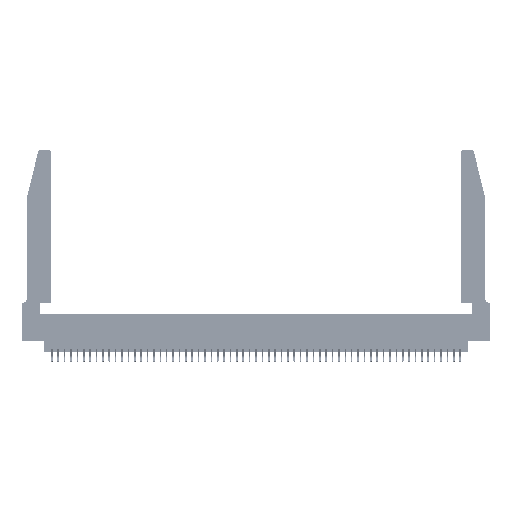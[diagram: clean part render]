
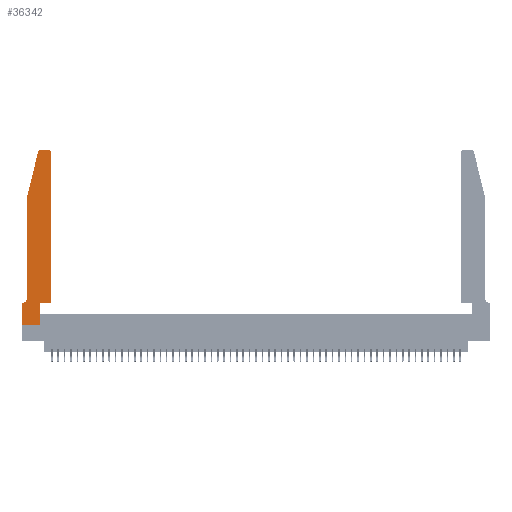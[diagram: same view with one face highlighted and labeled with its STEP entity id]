
A CAD part, top view. The second image highlights one B-rep face of the part: STEP entity #36342.
In plain terms, the highlighted planar face has unit normal (0, 0, 1).
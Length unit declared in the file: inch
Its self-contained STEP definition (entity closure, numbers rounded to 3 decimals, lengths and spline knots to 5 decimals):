
#1321 = DIRECTION ( 'NONE',  ( 0., 0., 1. ) ) ;
#2133 = DIRECTION ( 'NONE',  ( 0., -1., 0. ) ) ;
#2721 = VECTOR ( 'NONE', #9607, 39.37008 ) ;
#2754 = CIRCLE ( 'NONE', #3901, 0.03 ) ;
#3283 = VECTOR ( 'NONE', #47653, 39.37008 ) ;
#3629 = EDGE_CURVE ( 'NONE', #21828, #51516, #9514, .T. ) ;
#3901 = AXIS2_PLACEMENT_3D ( 'NONE', #47546, #23103, #51641 ) ;
#4372 = AXIS2_PLACEMENT_3D ( 'NONE', #9475, #1321, #30037 ) ;
#5228 = VERTEX_POINT ( 'NONE', #39480 ) ;
#5496 = ORIENTED_EDGE ( 'NONE', *, *, #44188, .T. ) ;
#5920 = VECTOR ( 'NONE', #51397, 39.37008 ) ;
#5972 = CARTESIAN_POINT ( 'NONE',  ( 0.4505, 0.35, 0.37 ) ) ;
#6263 = VERTEX_POINT ( 'NONE', #9507 ) ;
#6376 = CARTESIAN_POINT ( 'NONE',  ( 0.4505, 0.35, 0.37 ) ) ;
#7211 = DIRECTION ( 'NONE',  ( -1., 0., 0. ) ) ;
#8350 = ORIENTED_EDGE ( 'NONE', *, *, #20032, .T. ) ;
#8423 = ORIENTED_EDGE ( 'NONE', *, *, #27811, .T. ) ;
#8550 = CARTESIAN_POINT ( 'NONE',  ( 0.2865, 0.35, 0.37 ) ) ;
#8822 = VERTEX_POINT ( 'NONE', #28605 ) ;
#9288 = CARTESIAN_POINT ( 'NONE',  ( 0.4505, 0.35, 0.37 ) ) ;
#9475 = CARTESIAN_POINT ( 'NONE',  ( 0., 0.35, 0.37 ) ) ;
#9507 = CARTESIAN_POINT ( 'NONE',  ( 0.0755, 2., 0.37 ) ) ;
#9514 = LINE ( 'NONE', #35846, #39610 ) ;
#9607 = DIRECTION ( 'NONE',  ( -0.239, -0.971, 0. ) ) ;
#9857 = LINE ( 'NONE', #46904, #19444 ) ;
#11224 = LINE ( 'NONE', #5972, #42583 ) ;
#11283 = ORIENTED_EDGE ( 'NONE', *, *, #3629, .T. ) ;
#11904 = CARTESIAN_POINT ( 'NONE',  ( 0.284, 2.72, 0.37 ) ) ;
#12014 = CARTESIAN_POINT ( 'NONE',  ( 0.2865, 0.35, 0.37 ) ) ;
#14118 = EDGE_CURVE ( 'NONE', #51516, #5228, #30455, .T. ) ;
#14830 = VERTEX_POINT ( 'NONE', #24064 ) ;
#15171 = VECTOR ( 'NONE', #33038, 39.37008 ) ;
#16055 = DIRECTION ( 'NONE',  ( 1., 0., 0. ) ) ;
#16599 = VERTEX_POINT ( 'NONE', #46673 ) ;
#16742 = DIRECTION ( 'NONE',  ( 0., 0., -1. ) ) ;
#17714 = LINE ( 'NONE', #8550, #15171 ) ;
#18333 = DIRECTION ( 'NONE',  ( 1., 0., 0. ) ) ;
#19444 = VECTOR ( 'NONE', #2133, 39.37008 ) ;
#19560 = VECTOR ( 'NONE', #52471, 39.37008 ) ;
#20032 = EDGE_CURVE ( 'NONE', #5228, #8822, #33709, .T. ) ;
#20656 = AXIS2_PLACEMENT_3D ( 'NONE', #11904, #40543, #16055 ) ;
#21828 = VERTEX_POINT ( 'NONE', #37204 ) ;
#22852 = VECTOR ( 'NONE', #47160, 39.37008 ) ;
#23103 = DIRECTION ( 'NONE',  ( 0., 0., 1. ) ) ;
#23352 = AXIS2_PLACEMENT_3D ( 'NONE', #41251, #16742, #45304 ) ;
#23838 = CARTESIAN_POINT ( 'NONE',  ( 0.284, 2.75, 0.37 ) ) ;
#24064 = CARTESIAN_POINT ( 'NONE',  ( 0.4205, 2.75, 0.37 ) ) ;
#24875 = VERTEX_POINT ( 'NONE', #23838 ) ;
#27811 = EDGE_CURVE ( 'NONE', #24875, #16599, #34052, .T. ) ;
#28605 = CARTESIAN_POINT ( 'NONE',  ( 0.2865, 0., 0.37 ) ) ;
#28731 = VERTEX_POINT ( 'NONE', #38302 ) ;
#29203 = EDGE_CURVE ( 'NONE', #8822, #37995, #17714, .T. ) ;
#29231 = FACE_OUTER_BOUND ( 'NONE', #29858, .T. ) ;
#29858 = EDGE_LOOP ( 'NONE', ( #5496, #8423, #44074, #38468, #34824, #11283, #40611, #8350, #33218, #48213, #36288, #49190 ) ) ;
#30037 = DIRECTION ( 'NONE',  ( 1., 0., 0. ) ) ;
#30455 = LINE ( 'NONE', #40239, #19560 ) ;
#33038 = DIRECTION ( 'NONE',  ( 0., 1., 0. ) ) ;
#33218 = ORIENTED_EDGE ( 'NONE', *, *, #29203, .T. ) ;
#33709 = LINE ( 'NONE', #39010, #22852 ) ;
#33810 = CIRCLE ( 'NONE', #23352, 0.07 ) ;
#34052 = CIRCLE ( 'NONE', #20656, 0.03 ) ;
#34824 = ORIENTED_EDGE ( 'NONE', *, *, #49434, .T. ) ;
#35469 = LINE ( 'NONE', #46377, #2721 ) ;
#35846 = CARTESIAN_POINT ( 'NONE',  ( 0.0755, 0.35, 0.37 ) ) ;
#36033 = LINE ( 'NONE', #43595, #3283 ) ;
#36288 = ORIENTED_EDGE ( 'NONE', *, *, #44132, .T. ) ;
#36342 = ADVANCED_FACE ( 'NONE', ( #29231 ), #50357, .T. ) ;
#36701 = CARTESIAN_POINT ( 'NONE',  ( 0., 0.35, 0.37 ) ) ;
#37174 = EDGE_CURVE ( 'NONE', #37995, #43901, #11224, .T. ) ;
#37204 = CARTESIAN_POINT ( 'NONE',  ( 0.0055, 0.35, 0.37 ) ) ;
#37995 = VERTEX_POINT ( 'NONE', #12014 ) ;
#38302 = CARTESIAN_POINT ( 'NONE',  ( 0.4505, 2.72, 0.37 ) ) ;
#38468 = ORIENTED_EDGE ( 'NONE', *, *, #52598, .T. ) ;
#38602 = LINE ( 'NONE', #6376, #5920 ) ;
#39010 = CARTESIAN_POINT ( 'NONE',  ( 0., 0., 0.37 ) ) ;
#39480 = CARTESIAN_POINT ( 'NONE',  ( 0., 0., 0.37 ) ) ;
#39610 = VECTOR ( 'NONE', #7211, 39.37008 ) ;
#40239 = CARTESIAN_POINT ( 'NONE',  ( 0., 0., 0.37 ) ) ;
#40543 = DIRECTION ( 'NONE',  ( 0., 0., 1. ) ) ;
#40611 = ORIENTED_EDGE ( 'NONE', *, *, #14118, .T. ) ;
#41251 = CARTESIAN_POINT ( 'NONE',  ( 0.0055, 0.42, 0.37 ) ) ;
#41629 = CARTESIAN_POINT ( 'NONE',  ( 0.0755, 0.42, 0.37 ) ) ;
#41709 = VERTEX_POINT ( 'NONE', #41629 ) ;
#42583 = VECTOR ( 'NONE', #18333, 39.37008 ) ;
#43492 = EDGE_CURVE ( 'NONE', #28731, #14830, #2754, .T. ) ;
#43595 = CARTESIAN_POINT ( 'NONE',  ( 0.2605, 2.75, 0.37 ) ) ;
#43901 = VERTEX_POINT ( 'NONE', #9288 ) ;
#44074 = ORIENTED_EDGE ( 'NONE', *, *, #52480, .T. ) ;
#44132 = EDGE_CURVE ( 'NONE', #43901, #28731, #38602, .T. ) ;
#44188 = EDGE_CURVE ( 'NONE', #14830, #24875, #36033, .T. ) ;
#45304 = DIRECTION ( 'NONE',  ( -1., 0., 0. ) ) ;
#46377 = CARTESIAN_POINT ( 'NONE',  ( 0.0755, 2., 0.37 ) ) ;
#46673 = CARTESIAN_POINT ( 'NONE',  ( 0.25487, 2.72718, 0.37 ) ) ;
#46904 = CARTESIAN_POINT ( 'NONE',  ( 0.0755, 2., 0.37 ) ) ;
#47160 = DIRECTION ( 'NONE',  ( 1., 0., 0. ) ) ;
#47546 = CARTESIAN_POINT ( 'NONE',  ( 0.4205, 2.72, 0.37 ) ) ;
#47653 = DIRECTION ( 'NONE',  ( -1., 0., 0. ) ) ;
#48213 = ORIENTED_EDGE ( 'NONE', *, *, #37174, .T. ) ;
#49190 = ORIENTED_EDGE ( 'NONE', *, *, #43492, .T. ) ;
#49434 = EDGE_CURVE ( 'NONE', #41709, #21828, #33810, .T. ) ;
#50357 = PLANE ( 'NONE',  #4372 ) ;
#51397 = DIRECTION ( 'NONE',  ( 0., 1., 0. ) ) ;
#51516 = VERTEX_POINT ( 'NONE', #36701 ) ;
#51641 = DIRECTION ( 'NONE',  ( 1., 0., 0. ) ) ;
#52471 = DIRECTION ( 'NONE',  ( 0., -1., 0. ) ) ;
#52480 = EDGE_CURVE ( 'NONE', #16599, #6263, #35469, .T. ) ;
#52598 = EDGE_CURVE ( 'NONE', #6263, #41709, #9857, .T. ) ;
